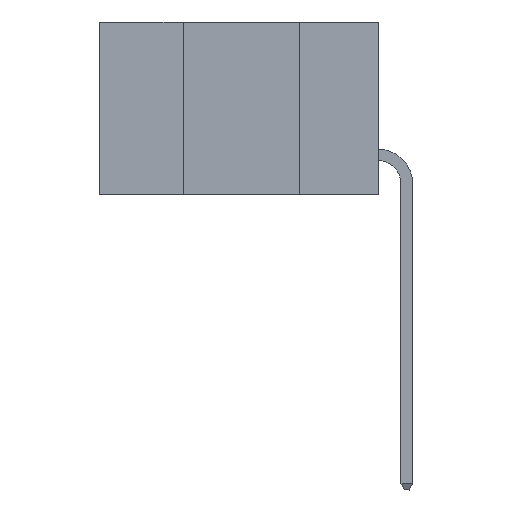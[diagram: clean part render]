
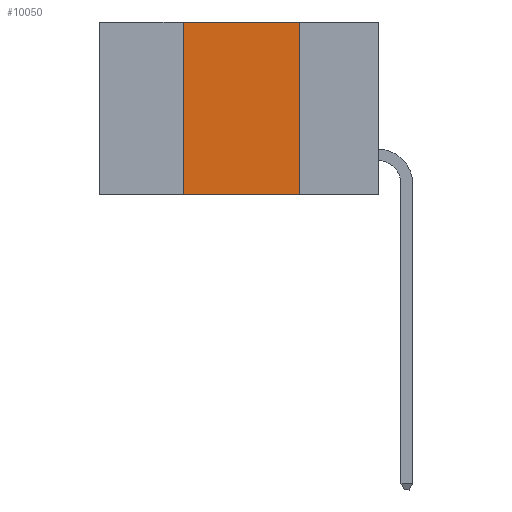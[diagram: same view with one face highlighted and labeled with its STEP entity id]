
A CAD part, left-side view. The second image highlights one B-rep face of the part: STEP entity #10050.
In plain terms, the highlighted planar face has unit normal (-1, 0, 0).
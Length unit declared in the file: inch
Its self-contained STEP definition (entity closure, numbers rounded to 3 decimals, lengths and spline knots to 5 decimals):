
#825 = LINE ( 'NONE', #13168, #7462 ) ;
#1569 = ORIENTED_EDGE ( 'NONE', *, *, #14988, .F. ) ;
#1770 = ORIENTED_EDGE ( 'NONE', *, *, #7495, .T. ) ;
#2030 = VERTEX_POINT ( 'NONE', #2198 ) ;
#2198 = CARTESIAN_POINT ( 'NONE',  ( 0., 0.17, -0.37 ) ) ;
#2505 = EDGE_CURVE ( 'NONE', #5018, #2030, #13856, .T. ) ;
#2683 = CARTESIAN_POINT ( 'NONE',  ( 0., 0.6, 0. ) ) ;
#3842 = EDGE_LOOP ( 'NONE', ( #14259, #1569, #12338, #1770 ) ) ;
#4001 = PLANE ( 'NONE',  #6888 ) ;
#5018 = VERTEX_POINT ( 'NONE', #15206 ) ;
#5166 = VECTOR ( 'NONE', #8984, 39.37008 ) ;
#5273 = EDGE_CURVE ( 'NONE', #11083, #8471, #825, .T. ) ;
#5683 = DIRECTION ( 'NONE',  ( 0., 0., -1. ) ) ;
#6888 = AXIS2_PLACEMENT_3D ( 'NONE', #2683, #15463, #12966 ) ;
#7462 = VECTOR ( 'NONE', #13128, 39.37008 ) ;
#7495 = EDGE_CURVE ( 'NONE', #11083, #2030, #9639, .T. ) ;
#7709 = CARTESIAN_POINT ( 'NONE',  ( 0., 0.6, 0. ) ) ;
#8005 = CARTESIAN_POINT ( 'NONE',  ( 0., 0.42, 0. ) ) ;
#8471 = VERTEX_POINT ( 'NONE', #8005 ) ;
#8984 = DIRECTION ( 'NONE',  ( 0., -1., 0. ) ) ;
#9639 = LINE ( 'NONE', #15317, #15960 ) ;
#10050 = ADVANCED_FACE ( 'NONE', ( #12903 ), #4001, .F. ) ;
#10505 = VECTOR ( 'NONE', #5683, 39.37008 ) ;
#11083 = VERTEX_POINT ( 'NONE', #11145 ) ;
#11145 = CARTESIAN_POINT ( 'NONE',  ( 0., 0.42, -0.37 ) ) ;
#12079 = CARTESIAN_POINT ( 'NONE',  ( 0., 0.17, 0. ) ) ;
#12338 = ORIENTED_EDGE ( 'NONE', *, *, #5273, .F. ) ;
#12903 = FACE_OUTER_BOUND ( 'NONE', #3842, .T. ) ;
#12966 = DIRECTION ( 'NONE',  ( 0., 0., -1. ) ) ;
#13128 = DIRECTION ( 'NONE',  ( 0., 0., 1. ) ) ;
#13168 = CARTESIAN_POINT ( 'NONE',  ( 0., 0.42, 0. ) ) ;
#13856 = LINE ( 'NONE', #12079, #10505 ) ;
#14259 = ORIENTED_EDGE ( 'NONE', *, *, #2505, .F. ) ;
#14988 = EDGE_CURVE ( 'NONE', #8471, #5018, #15341, .T. ) ;
#15206 = CARTESIAN_POINT ( 'NONE',  ( 0., 0.17, 0. ) ) ;
#15222 = DIRECTION ( 'NONE',  ( 0., -1., 0. ) ) ;
#15317 = CARTESIAN_POINT ( 'NONE',  ( 0., 0.6, -0.37 ) ) ;
#15341 = LINE ( 'NONE', #7709, #5166 ) ;
#15463 = DIRECTION ( 'NONE',  ( 1., 0., 0. ) ) ;
#15960 = VECTOR ( 'NONE', #15222, 39.37008 ) ;
